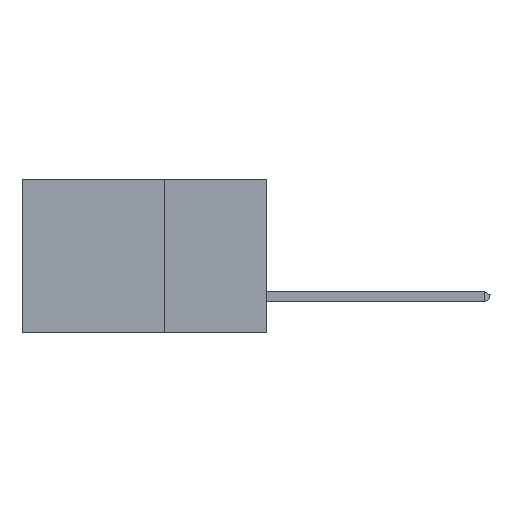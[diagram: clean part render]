
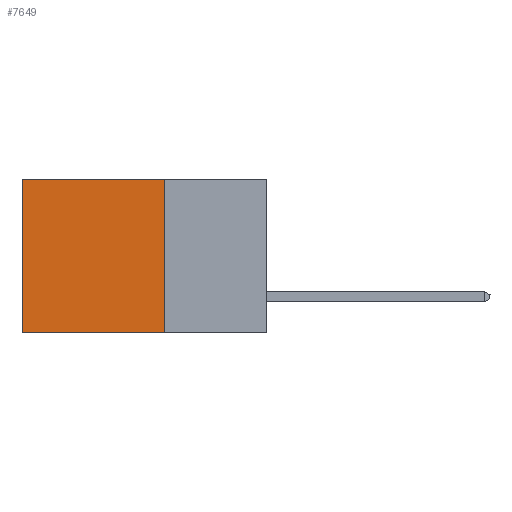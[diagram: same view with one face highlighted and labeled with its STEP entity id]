
A CAD part, left-side view. The second image highlights one B-rep face of the part: STEP entity #7649.
In plain terms, the highlighted planar face has unit normal (-1, 0, 0).
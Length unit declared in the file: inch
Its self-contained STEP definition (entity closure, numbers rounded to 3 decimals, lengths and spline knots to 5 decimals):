
#173 = VERTEX_POINT ( 'NONE', #15566 ) ;
#716 = VECTOR ( 'NONE', #9912, 39.37008 ) ;
#1708 = CARTESIAN_POINT ( 'NONE',  ( 0.2875, 0.6, -0.375 ) ) ;
#2003 = DIRECTION ( 'NONE',  ( 0., 1., 0. ) ) ;
#2670 = CARTESIAN_POINT ( 'NONE',  ( 0.2875, 0.6, -0.375 ) ) ;
#2745 = ORIENTED_EDGE ( 'NONE', *, *, #3533, .T. ) ;
#2870 = VECTOR ( 'NONE', #10950, 39.37008 ) ;
#3533 = EDGE_CURVE ( 'NONE', #173, #15736, #13544, .T. ) ;
#4115 = AXIS2_PLACEMENT_3D ( 'NONE', #8782, #5762, #12043 ) ;
#4274 = EDGE_CURVE ( 'NONE', #12713, #15736, #9421, .T. ) ;
#4549 = LINE ( 'NONE', #9383, #7975 ) ;
#5595 = EDGE_CURVE ( 'NONE', #12655, #12713, #7802, .T. ) ;
#5762 = DIRECTION ( 'NONE',  ( 1., 0., 0. ) ) ;
#5921 = CARTESIAN_POINT ( 'NONE',  ( 0.2875, 0.25, -0.375 ) ) ;
#6237 = FACE_OUTER_BOUND ( 'NONE', #15545, .T. ) ;
#7619 = PLANE ( 'NONE',  #4115 ) ;
#7649 = ADVANCED_FACE ( 'NONE', ( #6237 ), #7619, .F. ) ;
#7802 = LINE ( 'NONE', #5921, #2870 ) ;
#7975 = VECTOR ( 'NONE', #2003, 39.37008 ) ;
#8545 = CARTESIAN_POINT ( 'NONE',  ( 0.2875, 0.25, 0. ) ) ;
#8782 = CARTESIAN_POINT ( 'NONE',  ( 0.2875, 0.25, -0.375 ) ) ;
#8820 = ORIENTED_EDGE ( 'NONE', *, *, #15211, .T. ) ;
#9383 = CARTESIAN_POINT ( 'NONE',  ( 0.2875, 0.25, 0. ) ) ;
#9421 = LINE ( 'NONE', #16101, #716 ) ;
#9912 = DIRECTION ( 'NONE',  ( 0., 1., 0. ) ) ;
#10950 = DIRECTION ( 'NONE',  ( 0., 0., -1. ) ) ;
#12043 = DIRECTION ( 'NONE',  ( 0., 0., -1. ) ) ;
#12070 = ORIENTED_EDGE ( 'NONE', *, *, #5595, .F. ) ;
#12655 = VERTEX_POINT ( 'NONE', #8545 ) ;
#12713 = VERTEX_POINT ( 'NONE', #13633 ) ;
#12761 = VECTOR ( 'NONE', #14041, 39.37008 ) ;
#13544 = LINE ( 'NONE', #1708, #12761 ) ;
#13633 = CARTESIAN_POINT ( 'NONE',  ( 0.2875, 0.25, -0.375 ) ) ;
#13833 = ORIENTED_EDGE ( 'NONE', *, *, #4274, .F. ) ;
#14041 = DIRECTION ( 'NONE',  ( 0., 0., -1. ) ) ;
#15211 = EDGE_CURVE ( 'NONE', #12655, #173, #4549, .T. ) ;
#15545 = EDGE_LOOP ( 'NONE', ( #2745, #13833, #12070, #8820 ) ) ;
#15566 = CARTESIAN_POINT ( 'NONE',  ( 0.2875, 0.6, 0. ) ) ;
#15736 = VERTEX_POINT ( 'NONE', #2670 ) ;
#16101 = CARTESIAN_POINT ( 'NONE',  ( 0.2875, 0.25, -0.375 ) ) ;
